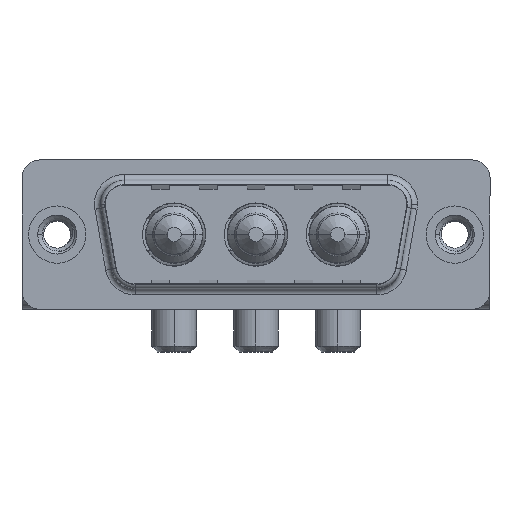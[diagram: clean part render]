
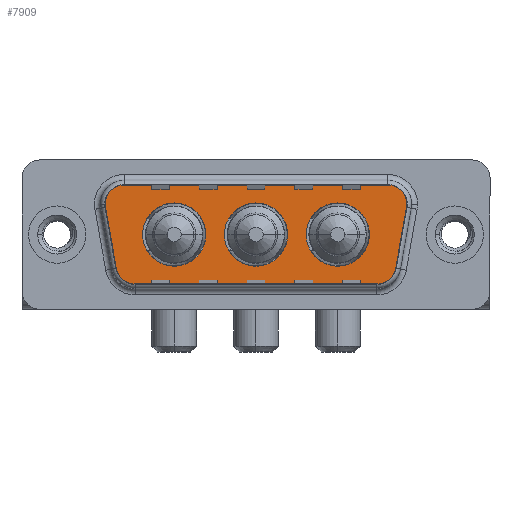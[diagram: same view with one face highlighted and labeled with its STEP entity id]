
A CAD part, top view. The second image highlights one B-rep face of the part: STEP entity #7909.
In plain terms, the highlighted planar face has unit normal (0, 0, 1).
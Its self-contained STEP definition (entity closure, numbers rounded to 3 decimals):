
#40 = DIRECTION ( 'NONE',  ( 0.174, -0.985, 0. ) ) ;
#60 = EDGE_CURVE ( 'NONE', #1815, #4023, #2140, .T. ) ;
#66 = CARTESIAN_POINT ( 'NONE',  ( 27.889, 4.9, 0. ) ) ;
#175 = AXIS2_PLACEMENT_3D ( 'NONE', #6840, #10311, #8078 ) ;
#228 = EDGE_CURVE ( 'NONE', #10725, #9716, #7254, .T. ) ;
#349 = DIRECTION ( 'NONE',  ( 1., 0., 0. ) ) ;
#375 = FACE_BOUND ( 'NONE', #1261, .T. ) ;
#414 = EDGE_CURVE ( 'NONE', #5974, #10725, #956, .T. ) ;
#507 = CARTESIAN_POINT ( 'NONE',  ( 26.866, -2.9, 0. ) ) ;
#589 = AXIS2_PLACEMENT_3D ( 'NONE', #1963, #7349, #8517 ) ;
#650 = CARTESIAN_POINT ( 'NONE',  ( 26.15, 0., 0. ) ) ;
#697 = DIRECTION ( 'NONE',  ( 0., 0., 1. ) ) ;
#762 = DIRECTION ( 'NONE',  ( -1., 0., 0. ) ) ;
#765 = DIRECTION ( 'NONE',  ( -1., 0., 0. ) ) ;
#789 = EDGE_CURVE ( 'NONE', #3427, #13657, #3181, .T. ) ;
#956 = LINE ( 'NONE', #12831, #6587 ) ;
#977 = CARTESIAN_POINT ( 'NONE',  ( 7.15, 0., 0. ) ) ;
#1138 = ORIENTED_EDGE ( 'NONE', *, *, #7374, .F. ) ;
#1243 = DIRECTION ( 'NONE',  ( -1., 0., 0. ) ) ;
#1261 = EDGE_LOOP ( 'NONE', ( #8434, #12660 ) ) ;
#1305 = LINE ( 'NONE', #11788, #7153 ) ;
#1795 = EDGE_LOOP ( 'NONE', ( #11187, #4743 ) ) ;
#1815 = VERTEX_POINT ( 'NONE', #977 ) ;
#1963 = CARTESIAN_POINT ( 'NONE',  ( 26.866, -2.9, 0. ) ) ;
#2140 = CIRCLE ( 'NONE', #3706, 2.65 ) ;
#2437 = AXIS2_PLACEMENT_3D ( 'NONE', #8486, #4242, #10710 ) ;
#2446 = AXIS2_PLACEMENT_3D ( 'NONE', #9224, #4841, #765 ) ;
#2501 = EDGE_CURVE ( 'NONE', #8280, #10939, #9471, .T. ) ;
#2507 = ORIENTED_EDGE ( 'NONE', *, *, #8479, .T. ) ;
#2600 = DIRECTION ( 'NONE',  ( 1., 0., 0. ) ) ;
#2663 = CARTESIAN_POINT ( 'NONE',  ( 6.434, -2.9, 0. ) ) ;
#2742 = CARTESIAN_POINT ( 'NONE',  ( 12.45, 0., 0. ) ) ;
#2984 = DIRECTION ( 'NONE',  ( 0., 0., 1. ) ) ;
#3181 = CIRCLE ( 'NONE', #10302, 2.65 ) ;
#3216 = CARTESIAN_POINT ( 'NONE',  ( 27.889, 2.9, 0. ) ) ;
#3427 = VERTEX_POINT ( 'NONE', #8965 ) ;
#3706 = AXIS2_PLACEMENT_3D ( 'NONE', #6599, #7766, #349 ) ;
#3999 = CIRCLE ( 'NONE', #175, 2.65 ) ;
#4023 = VERTEX_POINT ( 'NONE', #2742 ) ;
#4038 = DIRECTION ( 'NONE',  ( 1., 0., 0. ) ) ;
#4201 = DIRECTION ( 'NONE',  ( 0., 0., 1. ) ) ;
#4242 = DIRECTION ( 'NONE',  ( 0., 0., 1. ) ) ;
#4313 = ORIENTED_EDGE ( 'NONE', *, *, #228, .T. ) ;
#4398 = DIRECTION ( 'NONE',  ( 1., 0., 0. ) ) ;
#4510 = AXIS2_PLACEMENT_3D ( 'NONE', #6037, #697, #2600 ) ;
#4513 = CARTESIAN_POINT ( 'NONE',  ( 6.434, -4.9, 0. ) ) ;
#4652 = AXIS2_PLACEMENT_3D ( 'NONE', #11815, #11881, #9854 ) ;
#4664 = FACE_OUTER_BOUND ( 'NONE', #10901, .T. ) ;
#4700 = CARTESIAN_POINT ( 'NONE',  ( 14., 0., 0. ) ) ;
#4743 = ORIENTED_EDGE ( 'NONE', *, *, #2501, .F. ) ;
#4841 = DIRECTION ( 'NONE',  ( 0., 0., 1. ) ) ;
#4960 = CARTESIAN_POINT ( 'NONE',  ( 26.866, -4.9, 0. ) ) ;
#5145 = CIRCLE ( 'NONE', #2446, 2. ) ;
#5393 = CIRCLE ( 'NONE', #4510, 2.65 ) ;
#5539 = VECTOR ( 'NONE', #13631, 1000. ) ;
#5749 = DIRECTION ( 'NONE',  ( -1., 0., 0. ) ) ;
#5839 = FACE_BOUND ( 'NONE', #7613, .T. ) ;
#5974 = VERTEX_POINT ( 'NONE', #8021 ) ;
#5990 = DIRECTION ( 'NONE',  ( 1., 0., 0. ) ) ;
#6037 = CARTESIAN_POINT ( 'NONE',  ( 16.65, 0., 0. ) ) ;
#6093 = LINE ( 'NONE', #10330, #8658 ) ;
#6133 = EDGE_CURVE ( 'NONE', #7468, #8833, #9762, .T. ) ;
#6328 = CARTESIAN_POINT ( 'NONE',  ( 5.411, 4.9, 0. ) ) ;
#6330 = ORIENTED_EDGE ( 'NONE', *, *, #9486, .T. ) ;
#6380 = EDGE_CURVE ( 'NONE', #8833, #13129, #12168, .T. ) ;
#6587 = VECTOR ( 'NONE', #40, 1000. ) ;
#6599 = CARTESIAN_POINT ( 'NONE',  ( 9.8, 0., 0. ) ) ;
#6637 = EDGE_CURVE ( 'NONE', #4023, #1815, #11095, .T. ) ;
#6683 = VERTEX_POINT ( 'NONE', #66 ) ;
#6695 = FACE_BOUND ( 'NONE', #1795, .T. ) ;
#6840 = CARTESIAN_POINT ( 'NONE',  ( 23.5, 0., 0. ) ) ;
#6872 = CARTESIAN_POINT ( 'NONE',  ( 29.859, 2.553, 0. ) ) ;
#6929 = DIRECTION ( 'NONE',  ( 0., 0., 1. ) ) ;
#7114 = EDGE_CURVE ( 'NONE', #12248, #6683, #9991, .T. ) ;
#7153 = VECTOR ( 'NONE', #4398, 1000. ) ;
#7254 = CIRCLE ( 'NONE', #10803, 2. ) ;
#7265 = CARTESIAN_POINT ( 'NONE',  ( 28.836, -3.247, 0. ) ) ;
#7349 = DIRECTION ( 'NONE',  ( 0., 0., 1. ) ) ;
#7374 = EDGE_CURVE ( 'NONE', #13657, #3427, #3999, .T. ) ;
#7468 = VERTEX_POINT ( 'NONE', #4960 ) ;
#7496 = ORIENTED_EDGE ( 'NONE', *, *, #414, .T. ) ;
#7555 = AXIS2_PLACEMENT_3D ( 'NONE', #3216, #4201, #1243 ) ;
#7613 = EDGE_LOOP ( 'NONE', ( #1138, #9497 ) ) ;
#7766 = DIRECTION ( 'NONE',  ( 0., 0., 1. ) ) ;
#7909 = ADVANCED_FACE ( 'NONE', ( #6695, #5839, #375, #4664 ), #10082, .T. ) ;
#8021 = CARTESIAN_POINT ( 'NONE',  ( 3.441, 2.553, 0. ) ) ;
#8053 = ORIENTED_EDGE ( 'NONE', *, *, #6133, .T. ) ;
#8078 = DIRECTION ( 'NONE',  ( 1., 0., 0. ) ) ;
#8145 = CARTESIAN_POINT ( 'NONE',  ( 19.3, 0., 0. ) ) ;
#8280 = VERTEX_POINT ( 'NONE', #4700 ) ;
#8434 = ORIENTED_EDGE ( 'NONE', *, *, #6637, .F. ) ;
#8471 = ORIENTED_EDGE ( 'NONE', *, *, #10424, .T. ) ;
#8479 = EDGE_CURVE ( 'NONE', #6683, #10003, #6093, .T. ) ;
#8486 = CARTESIAN_POINT ( 'NONE',  ( 5.411, 2.9, 0. ) ) ;
#8517 = DIRECTION ( 'NONE',  ( 1., 0., 0. ) ) ;
#8541 = ORIENTED_EDGE ( 'NONE', *, *, #10290, .T. ) ;
#8658 = VECTOR ( 'NONE', #762, 1000. ) ;
#8679 = AXIS2_PLACEMENT_3D ( 'NONE', #507, #9038, #5990 ) ;
#8688 = CIRCLE ( 'NONE', #2437, 2. ) ;
#8833 = VERTEX_POINT ( 'NONE', #7265 ) ;
#8965 = CARTESIAN_POINT ( 'NONE',  ( 20.85, 0., 0. ) ) ;
#9038 = DIRECTION ( 'NONE',  ( 0., 0., 1. ) ) ;
#9118 = CARTESIAN_POINT ( 'NONE',  ( 23.5, 0., 0. ) ) ;
#9224 = CARTESIAN_POINT ( 'NONE',  ( 27.889, 2.9, 0. ) ) ;
#9471 = CIRCLE ( 'NONE', #10573, 2.65 ) ;
#9486 = EDGE_CURVE ( 'NONE', #10003, #5974, #8688, .T. ) ;
#9497 = ORIENTED_EDGE ( 'NONE', *, *, #789, .F. ) ;
#9553 = ORIENTED_EDGE ( 'NONE', *, *, #6380, .T. ) ;
#9716 = VERTEX_POINT ( 'NONE', #4513 ) ;
#9762 = CIRCLE ( 'NONE', #589, 2. ) ;
#9854 = DIRECTION ( 'NONE',  ( 1., 0., 0. ) ) ;
#9991 = CIRCLE ( 'NONE', #7555, 2. ) ;
#10003 = VERTEX_POINT ( 'NONE', #6328 ) ;
#10082 = PLANE ( 'NONE',  #8679 ) ;
#10290 = EDGE_CURVE ( 'NONE', #13129, #12248, #5145, .T. ) ;
#10302 = AXIS2_PLACEMENT_3D ( 'NONE', #9118, #2984, #4038 ) ;
#10311 = DIRECTION ( 'NONE',  ( 0., 0., 1. ) ) ;
#10330 = CARTESIAN_POINT ( 'NONE',  ( 5.411, 4.9, 0. ) ) ;
#10424 = EDGE_CURVE ( 'NONE', #9716, #7468, #1305, .T. ) ;
#10573 = AXIS2_PLACEMENT_3D ( 'NONE', #13753, #13682, #12629 ) ;
#10710 = DIRECTION ( 'NONE',  ( 1., 0., 0. ) ) ;
#10725 = VERTEX_POINT ( 'NONE', #11833 ) ;
#10803 = AXIS2_PLACEMENT_3D ( 'NONE', #2663, #6929, #5749 ) ;
#10901 = EDGE_LOOP ( 'NONE', ( #8053, #9553, #8541, #13788, #2507, #6330, #7496, #4313, #8471 ) ) ;
#10939 = VERTEX_POINT ( 'NONE', #8145 ) ;
#11095 = CIRCLE ( 'NONE', #4652, 2.65 ) ;
#11187 = ORIENTED_EDGE ( 'NONE', *, *, #11757, .F. ) ;
#11757 = EDGE_CURVE ( 'NONE', #10939, #8280, #5393, .T. ) ;
#11788 = CARTESIAN_POINT ( 'NONE',  ( 6.434, -4.9, 0. ) ) ;
#11815 = CARTESIAN_POINT ( 'NONE',  ( 9.8, 0., 0. ) ) ;
#11833 = CARTESIAN_POINT ( 'NONE',  ( 4.464, -3.247, 0. ) ) ;
#11881 = DIRECTION ( 'NONE',  ( 0., 0., 1. ) ) ;
#12168 = LINE ( 'NONE', #6872, #5539 ) ;
#12248 = VERTEX_POINT ( 'NONE', #12565 ) ;
#12565 = CARTESIAN_POINT ( 'NONE',  ( 29.889, 2.9, 0. ) ) ;
#12629 = DIRECTION ( 'NONE',  ( 1., 0., 0. ) ) ;
#12660 = ORIENTED_EDGE ( 'NONE', *, *, #60, .F. ) ;
#12831 = CARTESIAN_POINT ( 'NONE',  ( 3.441, 2.553, 0. ) ) ;
#13105 = CARTESIAN_POINT ( 'NONE',  ( 29.859, 2.553, 0. ) ) ;
#13129 = VERTEX_POINT ( 'NONE', #13105 ) ;
#13631 = DIRECTION ( 'NONE',  ( 0.174, 0.985, 0. ) ) ;
#13657 = VERTEX_POINT ( 'NONE', #650 ) ;
#13682 = DIRECTION ( 'NONE',  ( 0., 0., 1. ) ) ;
#13753 = CARTESIAN_POINT ( 'NONE',  ( 16.65, 0., 0. ) ) ;
#13788 = ORIENTED_EDGE ( 'NONE', *, *, #7114, .T. ) ;
